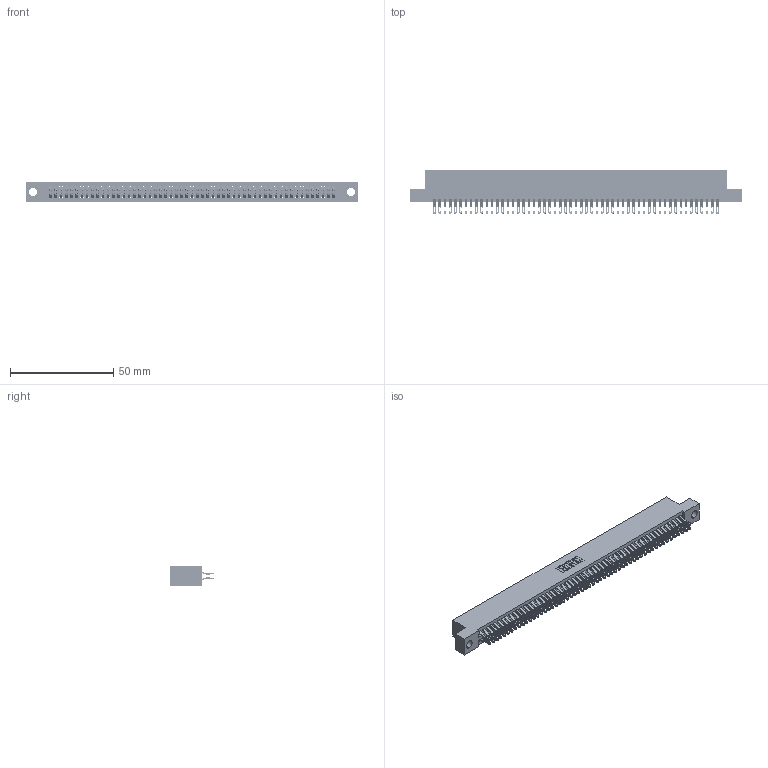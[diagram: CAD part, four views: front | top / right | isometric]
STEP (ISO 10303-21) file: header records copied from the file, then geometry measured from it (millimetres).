
FILE_DESCRIPTION (( 'STEP AP203' ), '1' );
FILE_NAME ('395-110-555-204.STEP', '2021-06-17T17:49:44', ( '' ), ( '' ), 'SwSTEP 2.0', 'SolidWorks 2020', '' );
FILE_SCHEMA (( 'CONFIG_CONTROL_DESIGN' ));
Length unit declared in the file: inch
Products named in the file (3): 395-110-555-204; 345 Part_Flush Mounting Lugs - 0.156 Dia-TI; 345-292-001_555 Tail
Assembly tree (111 placements, depth 2):
  395-110-555-204
    345 Part_Flush Mounting Lugs - 0.156 Dia-TI
    345-292-001_555 Tail  x110
Bounding box: 160.91 x 21.13 x 9.4 mm (x, y, z)
Volume: 15964.6 mm3; surface area: 24811.5 mm2
Topology: 111 solids, 111 shells, 6300 faces, 19847 edges, 13230 vertices
Faces by surface type: plane 3504, cylinder 2796
Entity records: 42149 total; most frequent: CARTESIAN_POINT 7092, ORIENTED_EDGE 6994, DIRECTION 6205, EDGE_CURVE 3497, VECTOR 3125, LINE 3125, VERTEX_POINT 2330, AXIS2_PLACEMENT_3D 1540
